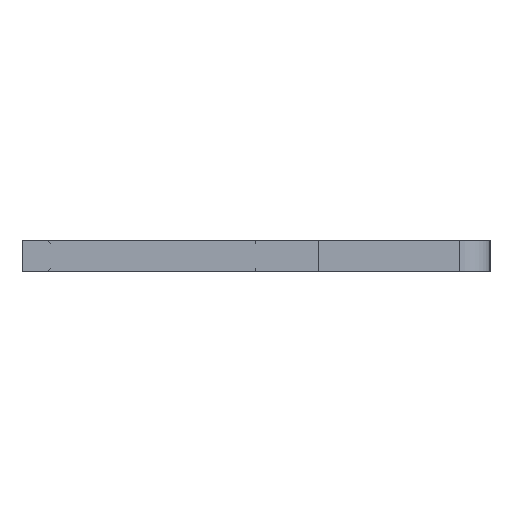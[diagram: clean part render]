
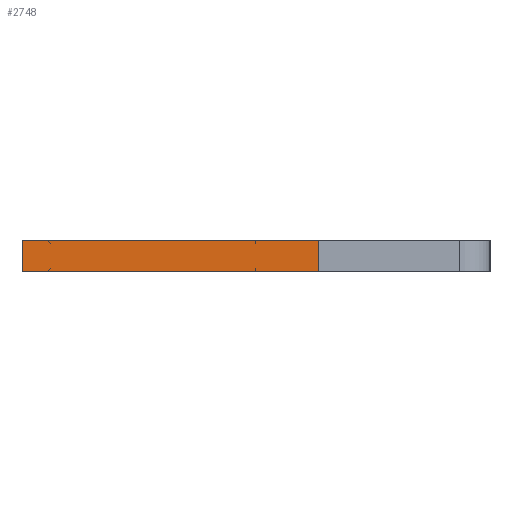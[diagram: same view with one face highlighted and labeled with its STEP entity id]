
A CAD part, left-side view. The second image highlights one B-rep face of the part: STEP entity #2748.
In plain terms, the highlighted face is planar.
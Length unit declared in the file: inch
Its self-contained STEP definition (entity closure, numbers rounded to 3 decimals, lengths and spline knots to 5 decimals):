
#114 = ORIENTED_EDGE ( 'NONE', *, *, #1920, .F. ) ;
#244 = EDGE_CURVE ( 'NONE', #1854, #1622, #1869, .T. ) ;
#450 = PLANE ( 'NONE',  #2323 ) ;
#455 = CARTESIAN_POINT ( 'NONE',  ( 0.01, -0.04, -0.04 ) ) ;
#613 = EDGE_CURVE ( 'NONE', #2764, #2660, #2483, .T. ) ;
#749 = CARTESIAN_POINT ( 'NONE',  ( 0.01, 0.15, -0.04 ) ) ;
#839 = ORIENTED_EDGE ( 'NONE', *, *, #1961, .T. ) ;
#959 = CARTESIAN_POINT ( 'NONE',  ( 0.01, 0.15, -0.04 ) ) ;
#986 = CARTESIAN_POINT ( 'NONE',  ( 0.01, 0.15, -0.04 ) ) ;
#997 = VECTOR ( 'NONE', #2508, 39.37008 ) ;
#1063 = DIRECTION ( 'NONE',  ( -1., 0., 0. ) ) ;
#1085 = FACE_OUTER_BOUND ( 'NONE', #1534, .T. ) ;
#1088 = VECTOR ( 'NONE', #2102, 39.37008 ) ;
#1285 = VECTOR ( 'NONE', #2805, 39.37008 ) ;
#1435 = CARTESIAN_POINT ( 'NONE',  ( 0.01, 0.15, -0.04 ) ) ;
#1488 = CARTESIAN_POINT ( 'NONE',  ( -0.01, 0.15, -0.04 ) ) ;
#1534 = EDGE_LOOP ( 'NONE', ( #839, #2517, #114, #2299 ) ) ;
#1622 = VERTEX_POINT ( 'NONE', #2119 ) ;
#1693 = CARTESIAN_POINT ( 'NONE',  ( -0.01, 0.15, -0.04 ) ) ;
#1767 = DIRECTION ( 'NONE',  ( 1., 0., 0. ) ) ;
#1788 = DIRECTION ( 'NONE',  ( 0., 0., 1. ) ) ;
#1854 = VERTEX_POINT ( 'NONE', #2760 ) ;
#1869 = LINE ( 'NONE', #455, #1088 ) ;
#1920 = EDGE_CURVE ( 'NONE', #1854, #2764, #3370, .T. ) ;
#1961 = EDGE_CURVE ( 'NONE', #1622, #2660, #3033, .T. ) ;
#2102 = DIRECTION ( 'NONE',  ( -1., 0., 0. ) ) ;
#2119 = CARTESIAN_POINT ( 'NONE',  ( -0.01, -0.04, -0.04 ) ) ;
#2299 = ORIENTED_EDGE ( 'NONE', *, *, #244, .T. ) ;
#2323 = AXIS2_PLACEMENT_3D ( 'NONE', #959, #1788, #1767 ) ;
#2483 = LINE ( 'NONE', #749, #3287 ) ;
#2508 = DIRECTION ( 'NONE',  ( 0., 1., 0. ) ) ;
#2517 = ORIENTED_EDGE ( 'NONE', *, *, #613, .F. ) ;
#2660 = VERTEX_POINT ( 'NONE', #1488 ) ;
#2748 = ADVANCED_FACE ( 'NONE', ( #1085 ), #450, .F. ) ;
#2760 = CARTESIAN_POINT ( 'NONE',  ( 0.01, -0.04, -0.04 ) ) ;
#2764 = VERTEX_POINT ( 'NONE', #986 ) ;
#2805 = DIRECTION ( 'NONE',  ( 0., 1., 0. ) ) ;
#3033 = LINE ( 'NONE', #1693, #1285 ) ;
#3287 = VECTOR ( 'NONE', #1063, 39.37008 ) ;
#3370 = LINE ( 'NONE', #1435, #997 ) ;
